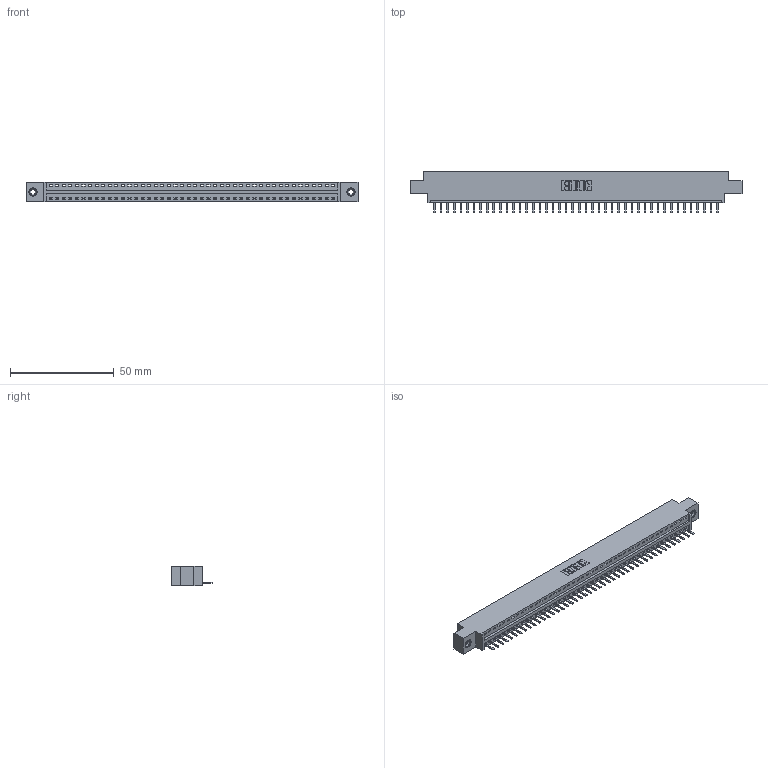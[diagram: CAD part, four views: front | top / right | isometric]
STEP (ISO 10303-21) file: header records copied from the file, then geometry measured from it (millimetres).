
FILE_DESCRIPTION (( 'STEP AP203' ), '1' );
FILE_NAME ('396-044-520-608.STEP', '2018-09-07T03:10:20', ( '' ), ( '' ), 'SwSTEP 2.0', 'SolidWorks 2016', '' );
FILE_SCHEMA (( 'CONFIG_CONTROL_DESIGN' ));
Length unit declared in the file: inch
Products named in the file (4): 396-044-520-608; 346 Part_0.170 Offset - 0.156 Dia-TI; 345-292-001_345-293-120; 345-250-001_345-250-003-102
Assembly tree (47 placements, depth 2):
  396-044-520-608
    346 Part_0.170 Offset - 0.156 Dia-TI
    345-292-001_345-293-120  x44
    345-250-001_345-250-003-102  x2
Bounding box: 160.27 x 20.02 x 9.4 mm (x, y, z)
Volume: 15067.9 mm3; surface area: 18614.1 mm2
Topology: 47 solids, 47 shells, 2914 faces, 8573 edges, 5590 vertices
Faces by surface type: plane 1960, cylinder 938, cone 12, torus 4
Entity records: 28470 total; most frequent: CARTESIAN_POINT 4875, ORIENTED_EDGE 4834, DIRECTION 4311, EDGE_CURVE 2417, LINE 2085, VECTOR 2085, VERTEX_POINT 1604, AXIS2_PLACEMENT_3D 1113
